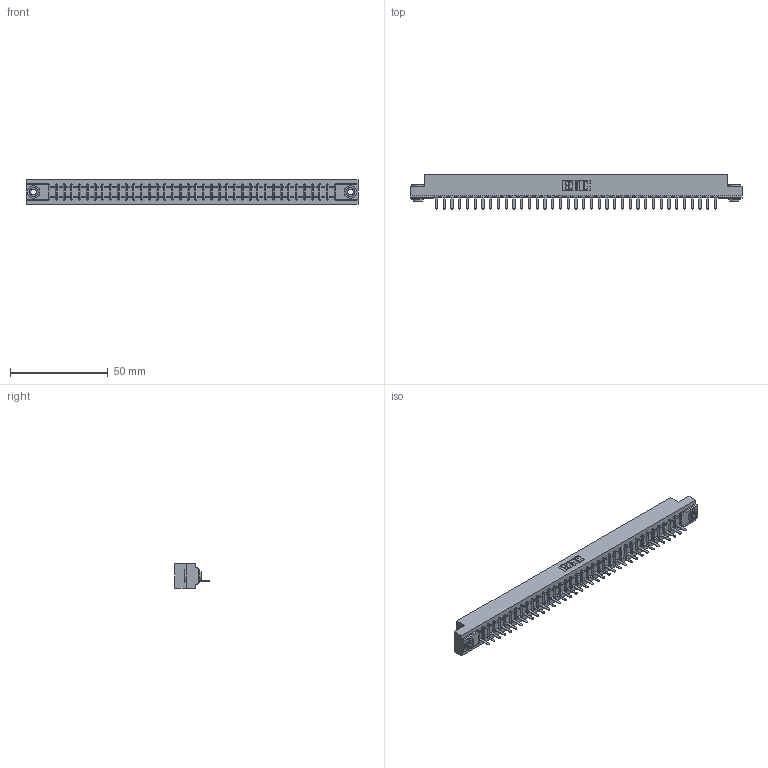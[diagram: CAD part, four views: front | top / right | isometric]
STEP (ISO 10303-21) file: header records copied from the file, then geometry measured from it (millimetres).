
FILE_DESCRIPTION (( 'STEP AP203' ), '1' );
FILE_NAME ('357-037-421-103.STEP', '2020-10-02T19:18:40', ( '' ), ( '' ), 'SwSTEP 2.0', 'SolidWorks 2020', '' );
FILE_SCHEMA (( 'CONFIG_CONTROL_DESIGN' ));
Length unit declared in the file: inch
Products named in the file (4): 345-250-002_345-250-002-102; 307 Part_.156 Dia Mounting Holes; 357-037-421-103; 307-290-002_521
Assembly tree (40 placements, depth 2):
  357-037-421-103
    307 Part_.156 Dia Mounting Holes
    307-290-002_521  x37
    345-250-002_345-250-002-102  x2
Bounding box: 169.62 x 17.42 x 12.7 mm (x, y, z)
Volume: 18117.8 mm3; surface area: 22926.5 mm2
Topology: 40 solids, 40 shells, 2946 faces, 9019 edges, 5906 vertices
Faces by surface type: plane 1759, cylinder 1103, sphere 76, cone 8
Entity records: 34119 total; most frequent: CARTESIAN_POINT 5733, ORIENTED_EDGE 5714, DIRECTION 5587, EDGE_CURVE 2857, VECTOR 2179, LINE 2179, VERTEX_POINT 1850, AXIS2_PLACEMENT_3D 1704
